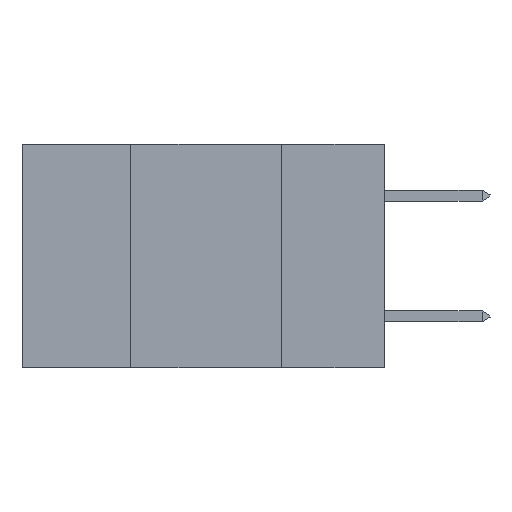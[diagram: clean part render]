
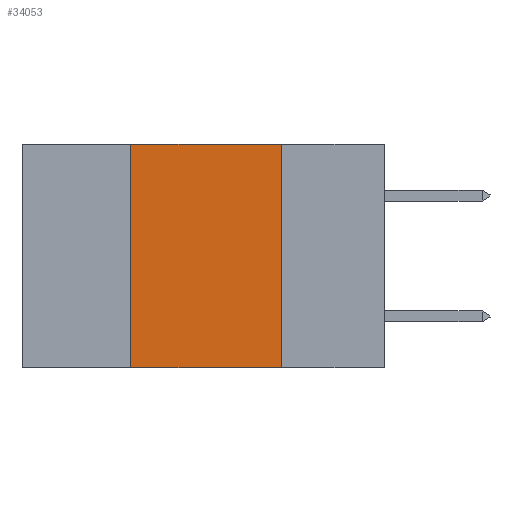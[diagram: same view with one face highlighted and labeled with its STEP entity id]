
A CAD part, left-side view. The second image highlights one B-rep face of the part: STEP entity #34053.
In plain terms, the highlighted planar face has unit normal (-1, 0, 0).
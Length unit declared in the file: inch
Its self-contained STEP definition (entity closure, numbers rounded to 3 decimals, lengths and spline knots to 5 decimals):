
#310 = VERTEX_POINT ( 'NONE', #25137 ) ;
#1177 = EDGE_CURVE ( 'NONE', #9303, #24807, #17556, .T. ) ;
#2627 = LINE ( 'NONE', #21800, #35217 ) ;
#3087 = CARTESIAN_POINT ( 'NONE',  ( 0., 0.6, 0. ) ) ;
#6252 = VERTEX_POINT ( 'NONE', #10853 ) ;
#8049 = EDGE_CURVE ( 'NONE', #6252, #24807, #8160, .T. ) ;
#8160 = LINE ( 'NONE', #28762, #15655 ) ;
#9159 = VECTOR ( 'NONE', #34654, 39.37008 ) ;
#9160 = AXIS2_PLACEMENT_3D ( 'NONE', #3087, #22840, #34363 ) ;
#9214 = CARTESIAN_POINT ( 'NONE',  ( 0., 0.17, 0. ) ) ;
#9303 = VERTEX_POINT ( 'NONE', #9214 ) ;
#10563 = EDGE_CURVE ( 'NONE', #6252, #310, #15051, .T. ) ;
#10853 = CARTESIAN_POINT ( 'NONE',  ( 0., 0.42, -0.37 ) ) ;
#14182 = PLANE ( 'NONE',  #9160 ) ;
#15051 = LINE ( 'NONE', #22319, #32759 ) ;
#15329 = CARTESIAN_POINT ( 'NONE',  ( 0., 0.17, 0. ) ) ;
#15655 = VECTOR ( 'NONE', #17503, 39.37008 ) ;
#16500 = EDGE_LOOP ( 'NONE', ( #24097, #28798, #20038, #21218 ) ) ;
#17503 = DIRECTION ( 'NONE',  ( 0., -1., 0. ) ) ;
#17556 = LINE ( 'NONE', #15329, #9159 ) ;
#18496 = FACE_OUTER_BOUND ( 'NONE', #16500, .T. ) ;
#20038 = ORIENTED_EDGE ( 'NONE', *, *, #10563, .F. ) ;
#21218 = ORIENTED_EDGE ( 'NONE', *, *, #8049, .T. ) ;
#21800 = CARTESIAN_POINT ( 'NONE',  ( 0., 0.6, 0. ) ) ;
#22319 = CARTESIAN_POINT ( 'NONE',  ( 0., 0.42, 0. ) ) ;
#22840 = DIRECTION ( 'NONE',  ( 1., 0., 0. ) ) ;
#24097 = ORIENTED_EDGE ( 'NONE', *, *, #1177, .F. ) ;
#24807 = VERTEX_POINT ( 'NONE', #25816 ) ;
#25137 = CARTESIAN_POINT ( 'NONE',  ( 0., 0.42, 0. ) ) ;
#25816 = CARTESIAN_POINT ( 'NONE',  ( 0., 0.17, -0.37 ) ) ;
#28762 = CARTESIAN_POINT ( 'NONE',  ( 0., 0.6, -0.37 ) ) ;
#28798 = ORIENTED_EDGE ( 'NONE', *, *, #33985, .F. ) ;
#32759 = VECTOR ( 'NONE', #33595, 39.37008 ) ;
#33595 = DIRECTION ( 'NONE',  ( 0., 0., 1. ) ) ;
#33985 = EDGE_CURVE ( 'NONE', #310, #9303, #2627, .T. ) ;
#34053 = ADVANCED_FACE ( 'NONE', ( #18496 ), #14182, .F. ) ;
#34363 = DIRECTION ( 'NONE',  ( 0., 0., -1. ) ) ;
#34654 = DIRECTION ( 'NONE',  ( 0., 0., -1. ) ) ;
#35217 = VECTOR ( 'NONE', #36132, 39.37008 ) ;
#36132 = DIRECTION ( 'NONE',  ( 0., -1., 0. ) ) ;
